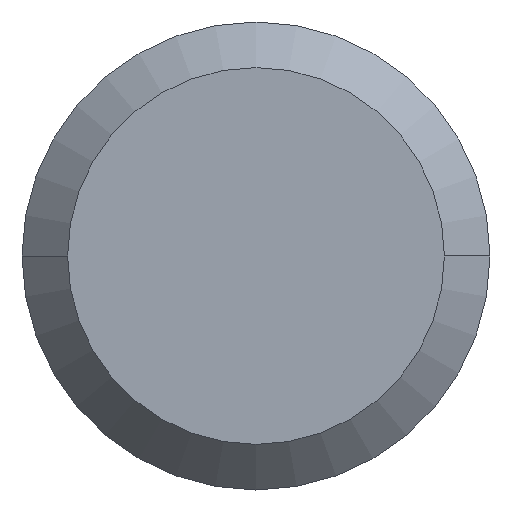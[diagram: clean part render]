
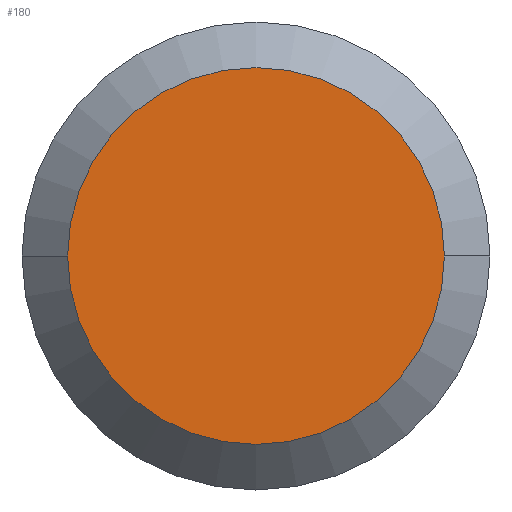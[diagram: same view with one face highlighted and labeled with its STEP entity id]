
A CAD part, left-side view. The second image highlights one B-rep face of the part: STEP entity #180.
In plain terms, the highlighted planar face has unit normal (-1, 0, 0).
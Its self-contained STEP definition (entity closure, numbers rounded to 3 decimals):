
#8 = CIRCLE ( 'NONE', #317, 1.575 ) ;
#25 = AXIS2_PLACEMENT_3D ( 'NONE', #547, #556, #167 ) ;
#41 = CARTESIAN_POINT ( 'NONE',  ( 0., 0., 0. ) ) ;
#57 = ORIENTED_EDGE ( 'NONE', *, *, #207, .F. ) ;
#108 = DIRECTION ( 'NONE',  ( 1., 0., 0. ) ) ;
#123 = CIRCLE ( 'NONE', #210, 1.575 ) ;
#167 = DIRECTION ( 'NONE',  ( 0., 0., 1. ) ) ;
#180 = ADVANCED_FACE ( 'NONE', ( #683 ), #803, .T. ) ;
#198 = EDGE_CURVE ( 'NONE', #462, #209, #8, .T. ) ;
#207 = EDGE_CURVE ( 'NONE', #209, #462, #123, .T. ) ;
#209 = VERTEX_POINT ( 'NONE', #807 ) ;
#210 = AXIS2_PLACEMENT_3D ( 'NONE', #236, #364, #736 ) ;
#236 = CARTESIAN_POINT ( 'NONE',  ( 0., 0., 0. ) ) ;
#284 = EDGE_LOOP ( 'NONE', ( #327, #57 ) ) ;
#317 = AXIS2_PLACEMENT_3D ( 'NONE', #41, #108, #488 ) ;
#327 = ORIENTED_EDGE ( 'NONE', *, *, #198, .F. ) ;
#364 = DIRECTION ( 'NONE',  ( 1., 0., 0. ) ) ;
#462 = VERTEX_POINT ( 'NONE', #676 ) ;
#488 = DIRECTION ( 'NONE',  ( 0., 0., -1. ) ) ;
#547 = CARTESIAN_POINT ( 'NONE',  ( 0., 1.575, 0. ) ) ;
#556 = DIRECTION ( 'NONE',  ( -1., 0., 0. ) ) ;
#676 = CARTESIAN_POINT ( 'NONE',  ( 0., 1.575, 0. ) ) ;
#683 = FACE_OUTER_BOUND ( 'NONE', #284, .T. ) ;
#736 = DIRECTION ( 'NONE',  ( 0., 0., -1. ) ) ;
#803 = PLANE ( 'NONE',  #25 ) ;
#807 = CARTESIAN_POINT ( 'NONE',  ( 0., -1.575, 0. ) ) ;
